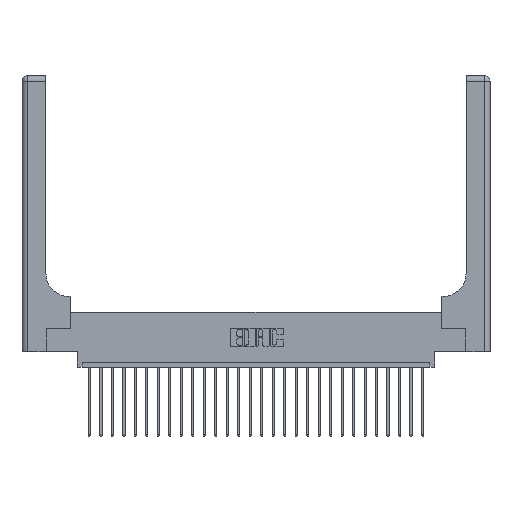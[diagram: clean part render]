
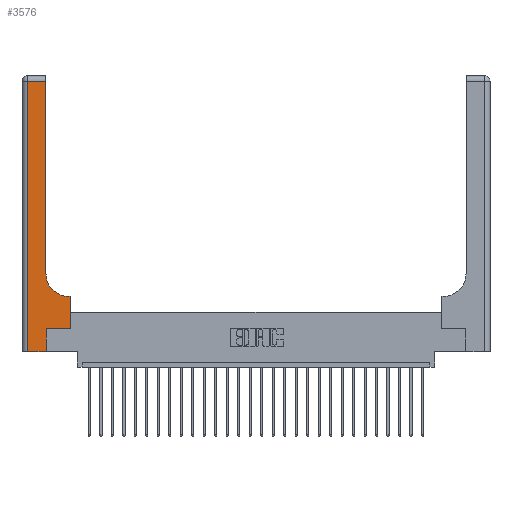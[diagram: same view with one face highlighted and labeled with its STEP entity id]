
A CAD part, top view. The second image highlights one B-rep face of the part: STEP entity #3576.
In plain terms, the highlighted planar face has unit normal (0, 0, 1).
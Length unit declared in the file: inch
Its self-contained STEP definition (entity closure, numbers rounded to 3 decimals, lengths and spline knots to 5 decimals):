
#34 = DIRECTION ( 'NONE',  ( 0., 1., 0. ) ) ;
#475 = CARTESIAN_POINT ( 'NONE',  ( 0.528, 0.6, 0.37 ) ) ;
#1078 = LINE ( 'NONE', #7088, #8481 ) ;
#1235 = CARTESIAN_POINT ( 'NONE',  ( 0.06, 0., 0.37 ) ) ;
#1566 = DIRECTION ( 'NONE',  ( 0., 1., 0. ) ) ;
#2003 = LINE ( 'NONE', #10008, #23893 ) ;
#2160 = LINE ( 'NONE', #25850, #18986 ) ;
#2378 = VERTEX_POINT ( 'NONE', #25483 ) ;
#2730 = CARTESIAN_POINT ( 'NONE',  ( 0.265, 0.25, 0.37 ) ) ;
#3051 = ORIENTED_EDGE ( 'NONE', *, *, #6747, .T. ) ;
#3400 = EDGE_CURVE ( 'NONE', #22921, #23080, #2003, .T. ) ;
#3416 = DIRECTION ( 'NONE',  ( -1., 0., 0. ) ) ;
#3576 = ADVANCED_FACE ( 'NONE', ( #13535 ), #21185, .F. ) ;
#3628 = ORIENTED_EDGE ( 'NONE', *, *, #8957, .T. ) ;
#4879 = DIRECTION ( 'NONE',  ( -1., 0., 0. ) ) ;
#4961 = EDGE_CURVE ( 'NONE', #23080, #18272, #8007, .T. ) ;
#4975 = LINE ( 'NONE', #6404, #18068 ) ;
#6404 = CARTESIAN_POINT ( 'NONE',  ( 0.265, 0., 0.37 ) ) ;
#6747 = EDGE_CURVE ( 'NONE', #2378, #25460, #12747, .T. ) ;
#6810 = CARTESIAN_POINT ( 'NONE',  ( 0.06, 2.94, 0.37 ) ) ;
#7054 = DIRECTION ( 'NONE',  ( 1., 0., 0. ) ) ;
#7088 = CARTESIAN_POINT ( 'NONE',  ( 0., 2.94, 0.37 ) ) ;
#7235 = CARTESIAN_POINT ( 'NONE',  ( 0., 0., 0.37 ) ) ;
#7580 = ORIENTED_EDGE ( 'NONE', *, *, #3400, .T. ) ;
#7664 = CARTESIAN_POINT ( 'NONE',  ( 0.265, 0.25, 0.37 ) ) ;
#8007 = LINE ( 'NONE', #8141, #25127 ) ;
#8141 = CARTESIAN_POINT ( 'NONE',  ( 0.26, 0.6, 0.37 ) ) ;
#8360 = EDGE_CURVE ( 'NONE', #8677, #21287, #4975, .T. ) ;
#8481 = VECTOR ( 'NONE', #4879, 39.37008 ) ;
#8677 = VERTEX_POINT ( 'NONE', #20456 ) ;
#8957 = EDGE_CURVE ( 'NONE', #22868, #14162, #2160, .T. ) ;
#10008 = CARTESIAN_POINT ( 'NONE',  ( 0.528, 0.25, 0.37 ) ) ;
#10490 = ORIENTED_EDGE ( 'NONE', *, *, #21745, .T. ) ;
#10773 = DIRECTION ( 'NONE',  ( 0., 1., 0. ) ) ;
#11091 = VECTOR ( 'NONE', #19486, 39.37008 ) ;
#11330 = VECTOR ( 'NONE', #10773, 39.37008 ) ;
#11913 = ORIENTED_EDGE ( 'NONE', *, *, #25868, .T. ) ;
#12485 = CARTESIAN_POINT ( 'NONE',  ( 0.26, 3., 0.37 ) ) ;
#12747 = LINE ( 'NONE', #12485, #11330 ) ;
#13117 = DIRECTION ( 'NONE',  ( 0., 0., -1. ) ) ;
#13535 = FACE_OUTER_BOUND ( 'NONE', #20333, .T. ) ;
#14162 = VERTEX_POINT ( 'NONE', #1235 ) ;
#15124 = CARTESIAN_POINT ( 'NONE',  ( 0.51, 0.6, 0.37 ) ) ;
#15160 = EDGE_CURVE ( 'NONE', #21287, #22921, #25586, .T. ) ;
#15370 = CIRCLE ( 'NONE', #20838, 0.25 ) ;
#15384 = DIRECTION ( 'NONE',  ( 0., 0., -1. ) ) ;
#16693 = AXIS2_PLACEMENT_3D ( 'NONE', #19338, #15384, #3416 ) ;
#17242 = ORIENTED_EDGE ( 'NONE', *, *, #18219, .T. ) ;
#18068 = VECTOR ( 'NONE', #1566, 39.37008 ) ;
#18219 = EDGE_CURVE ( 'NONE', #25460, #22868, #1078, .T. ) ;
#18272 = VERTEX_POINT ( 'NONE', #15124 ) ;
#18986 = VECTOR ( 'NONE', #22145, 39.37008 ) ;
#19161 = ORIENTED_EDGE ( 'NONE', *, *, #4961, .T. ) ;
#19338 = CARTESIAN_POINT ( 'NONE',  ( 0., 3., 0.37 ) ) ;
#19486 = DIRECTION ( 'NONE',  ( 1., 0., 0. ) ) ;
#19679 = CARTESIAN_POINT ( 'NONE',  ( 0.528, 0.25, 0.37 ) ) ;
#20333 = EDGE_LOOP ( 'NONE', ( #3051, #17242, #3628, #10490, #23539, #22373, #7580, #19161, #11913 ) ) ;
#20456 = CARTESIAN_POINT ( 'NONE',  ( 0.265, 0., 0.37 ) ) ;
#20838 = AXIS2_PLACEMENT_3D ( 'NONE', #23011, #13117, #7054 ) ;
#21067 = VECTOR ( 'NONE', #21751, 39.37008 ) ;
#21185 = PLANE ( 'NONE',  #16693 ) ;
#21287 = VERTEX_POINT ( 'NONE', #2730 ) ;
#21745 = EDGE_CURVE ( 'NONE', #14162, #8677, #25290, .T. ) ;
#21751 = DIRECTION ( 'NONE',  ( 1., 0., 0. ) ) ;
#22145 = DIRECTION ( 'NONE',  ( 0., -1., 0. ) ) ;
#22373 = ORIENTED_EDGE ( 'NONE', *, *, #15160, .T. ) ;
#22868 = VERTEX_POINT ( 'NONE', #6810 ) ;
#22921 = VERTEX_POINT ( 'NONE', #19679 ) ;
#23011 = CARTESIAN_POINT ( 'NONE',  ( 0.51, 0.85, 0.37 ) ) ;
#23080 = VERTEX_POINT ( 'NONE', #475 ) ;
#23539 = ORIENTED_EDGE ( 'NONE', *, *, #8360, .T. ) ;
#23893 = VECTOR ( 'NONE', #34, 39.37008 ) ;
#24343 = DIRECTION ( 'NONE',  ( -1., 0., 0. ) ) ;
#25127 = VECTOR ( 'NONE', #24343, 39.37008 ) ;
#25290 = LINE ( 'NONE', #7235, #11091 ) ;
#25412 = CARTESIAN_POINT ( 'NONE',  ( 0.26, 2.94, 0.37 ) ) ;
#25460 = VERTEX_POINT ( 'NONE', #25412 ) ;
#25483 = CARTESIAN_POINT ( 'NONE',  ( 0.26, 0.85, 0.37 ) ) ;
#25586 = LINE ( 'NONE', #7664, #21067 ) ;
#25850 = CARTESIAN_POINT ( 'NONE',  ( 0.06, 3., 0.37 ) ) ;
#25868 = EDGE_CURVE ( 'NONE', #18272, #2378, #15370, .T. ) ;
